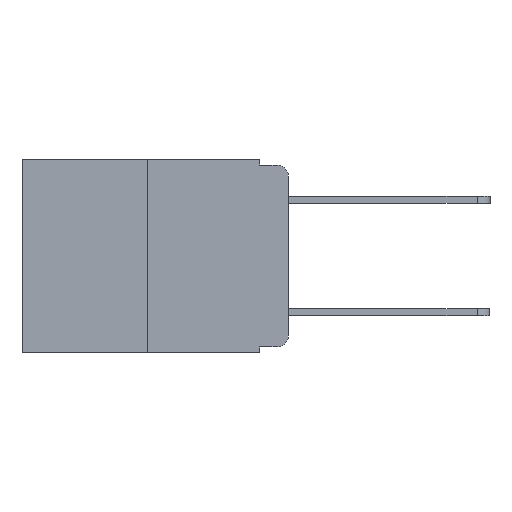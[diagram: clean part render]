
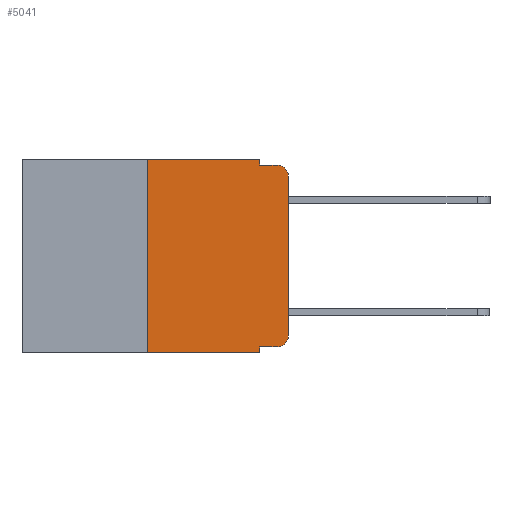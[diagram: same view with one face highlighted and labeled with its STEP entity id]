
A CAD part, left-side view. The second image highlights one B-rep face of the part: STEP entity #5041.
In plain terms, the highlighted planar face has unit normal (-1, 0, 0).
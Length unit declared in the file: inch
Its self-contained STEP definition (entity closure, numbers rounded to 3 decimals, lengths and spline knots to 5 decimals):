
#167 = LINE ( 'NONE', #6463, #14664 ) ;
#312 = CARTESIAN_POINT ( 'NONE',  ( 0., 0.25, 0. ) ) ;
#531 = DIRECTION ( 'NONE',  ( 0., 0., -1. ) ) ;
#774 = PLANE ( 'NONE',  #15957 ) ;
#1129 = LINE ( 'NONE', #14060, #8820 ) ;
#1146 = VECTOR ( 'NONE', #3862, 39.37008 ) ;
#1408 = LINE ( 'NONE', #12126, #12087 ) ;
#1503 = VERTEX_POINT ( 'NONE', #8934 ) ;
#1636 = VECTOR ( 'NONE', #7823, 39.37008 ) ;
#1720 = VECTOR ( 'NONE', #3331, 39.37008 ) ;
#1839 = AXIS2_PLACEMENT_3D ( 'NONE', #15441, #7893, #16526 ) ;
#1857 = CARTESIAN_POINT ( 'NONE',  ( 0., 0.02, -0.333 ) ) ;
#2173 = VERTEX_POINT ( 'NONE', #11022 ) ;
#2249 = CARTESIAN_POINT ( 'NONE',  ( 0., 0.473, 0. ) ) ;
#2266 = ORIENTED_EDGE ( 'NONE', *, *, #4326, .T. ) ;
#2307 = VERTEX_POINT ( 'NONE', #14927 ) ;
#2318 = DIRECTION ( 'NONE',  ( 1., 0., 0. ) ) ;
#2442 = VERTEX_POINT ( 'NONE', #15842 ) ;
#3135 = CARTESIAN_POINT ( 'NONE',  ( 0., 0.02, -0.03 ) ) ;
#3331 = DIRECTION ( 'NONE',  ( 0., 0., 1. ) ) ;
#3380 = ORIENTED_EDGE ( 'NONE', *, *, #4320, .F. ) ;
#3409 = CARTESIAN_POINT ( 'NONE',  ( 0., 0.051, 0. ) ) ;
#3502 = EDGE_CURVE ( 'NONE', #2173, #9221, #1408, .T. ) ;
#3862 = DIRECTION ( 'NONE',  ( 0., -1., 0. ) ) ;
#3949 = EDGE_CURVE ( 'NONE', #2442, #11313, #15726, .T. ) ;
#4259 = EDGE_CURVE ( 'NONE', #11148, #8178, #1129, .T. ) ;
#4266 = EDGE_CURVE ( 'NONE', #8178, #16630, #15002, .T. ) ;
#4288 = EDGE_CURVE ( 'NONE', #1503, #16630, #4806, .T. ) ;
#4294 = EDGE_CURVE ( 'NONE', #9221, #1503, #167, .T. ) ;
#4297 = EDGE_CURVE ( 'NONE', #2442, #2173, #11471, .T. ) ;
#4320 = EDGE_CURVE ( 'NONE', #2307, #11313, #13389, .T. ) ;
#4326 = EDGE_CURVE ( 'NONE', #2307, #8748, #13027, .T. ) ;
#4352 = EDGE_CURVE ( 'NONE', #8748, #11148, #16074, .T. ) ;
#4579 = DIRECTION ( 'NONE',  ( 0., 0., 1. ) ) ;
#4806 = LINE ( 'NONE', #8986, #7846 ) ;
#4826 = ORIENTED_EDGE ( 'NONE', *, *, #4297, .F. ) ;
#4951 = DIRECTION ( 'NONE',  ( 0., 0., -1. ) ) ;
#5041 = ADVANCED_FACE ( 'NONE', ( #9927 ), #774, .F. ) ;
#5173 = CARTESIAN_POINT ( 'NONE',  ( 0., 0.051, 0. ) ) ;
#5256 = ORIENTED_EDGE ( 'NONE', *, *, #4352, .T. ) ;
#5313 = EDGE_LOOP ( 'NONE', ( #12256, #17105, #15170, #11986, #13236, #4826, #5765, #3380, #2266, #5256 ) ) ;
#5765 = ORIENTED_EDGE ( 'NONE', *, *, #3949, .T. ) ;
#6463 = CARTESIAN_POINT ( 'NONE',  ( 0., 0.051, 0. ) ) ;
#6522 = DIRECTION ( 'NONE',  ( 0., 0., -1. ) ) ;
#7823 = DIRECTION ( 'NONE',  ( 0., -1., 0. ) ) ;
#7846 = VECTOR ( 'NONE', #15491, 39.37008 ) ;
#7893 = DIRECTION ( 'NONE',  ( -1., 0., 0. ) ) ;
#8178 = VERTEX_POINT ( 'NONE', #10207 ) ;
#8748 = VERTEX_POINT ( 'NONE', #1857 ) ;
#8820 = VECTOR ( 'NONE', #4579, 39.37008 ) ;
#8934 = CARTESIAN_POINT ( 'NONE',  ( 0., 0.051, -0.01 ) ) ;
#8986 = CARTESIAN_POINT ( 'NONE',  ( 0., 0.051, -0.01 ) ) ;
#9221 = VERTEX_POINT ( 'NONE', #5173 ) ;
#9366 = CARTESIAN_POINT ( 'NONE',  ( 0., 0.02, -0.01 ) ) ;
#9596 = DIRECTION ( 'NONE',  ( 0., -1., 0. ) ) ;
#9927 = FACE_OUTER_BOUND ( 'NONE', #5313, .T. ) ;
#10151 = VECTOR ( 'NONE', #6522, 39.37008 ) ;
#10207 = CARTESIAN_POINT ( 'NONE',  ( 0., 0., -0.03 ) ) ;
#10917 = CARTESIAN_POINT ( 'NONE',  ( 0., 0., -0.313 ) ) ;
#11022 = CARTESIAN_POINT ( 'NONE',  ( 0., 0.25, 0. ) ) ;
#11127 = AXIS2_PLACEMENT_3D ( 'NONE', #3135, #12976, #531 ) ;
#11148 = VERTEX_POINT ( 'NONE', #10917 ) ;
#11313 = VERTEX_POINT ( 'NONE', #12262 ) ;
#11471 = LINE ( 'NONE', #312, #1720 ) ;
#11986 = ORIENTED_EDGE ( 'NONE', *, *, #4294, .F. ) ;
#12054 = CARTESIAN_POINT ( 'NONE',  ( 0., 0.051, -0.333 ) ) ;
#12087 = VECTOR ( 'NONE', #9596, 39.37008 ) ;
#12126 = CARTESIAN_POINT ( 'NONE',  ( 0., 0.473, 0. ) ) ;
#12256 = ORIENTED_EDGE ( 'NONE', *, *, #4259, .T. ) ;
#12262 = CARTESIAN_POINT ( 'NONE',  ( 0., 0.051, -0.343 ) ) ;
#12385 = DIRECTION ( 'NONE',  ( 0., 0., -1. ) ) ;
#12754 = CARTESIAN_POINT ( 'NONE',  ( 0., 0.473, -0.343 ) ) ;
#12976 = DIRECTION ( 'NONE',  ( -1., 0., 0. ) ) ;
#13027 = LINE ( 'NONE', #12054, #1636 ) ;
#13236 = ORIENTED_EDGE ( 'NONE', *, *, #3502, .F. ) ;
#13389 = LINE ( 'NONE', #3409, #10151 ) ;
#14060 = CARTESIAN_POINT ( 'NONE',  ( 0., 0., 0. ) ) ;
#14664 = VECTOR ( 'NONE', #4951, 39.37008 ) ;
#14927 = CARTESIAN_POINT ( 'NONE',  ( 0., 0.051, -0.333 ) ) ;
#15002 = CIRCLE ( 'NONE', #11127, 0.02 ) ;
#15170 = ORIENTED_EDGE ( 'NONE', *, *, #4288, .F. ) ;
#15441 = CARTESIAN_POINT ( 'NONE',  ( 0., 0.02, -0.313 ) ) ;
#15491 = DIRECTION ( 'NONE',  ( 0., -1., 0. ) ) ;
#15726 = LINE ( 'NONE', #12754, #1146 ) ;
#15842 = CARTESIAN_POINT ( 'NONE',  ( 0., 0.25, -0.343 ) ) ;
#15957 = AXIS2_PLACEMENT_3D ( 'NONE', #2249, #2318, #12385 ) ;
#16074 = CIRCLE ( 'NONE', #1839, 0.02 ) ;
#16526 = DIRECTION ( 'NONE',  ( 0., 0., -1. ) ) ;
#16630 = VERTEX_POINT ( 'NONE', #9366 ) ;
#17105 = ORIENTED_EDGE ( 'NONE', *, *, #4266, .T. ) ;
